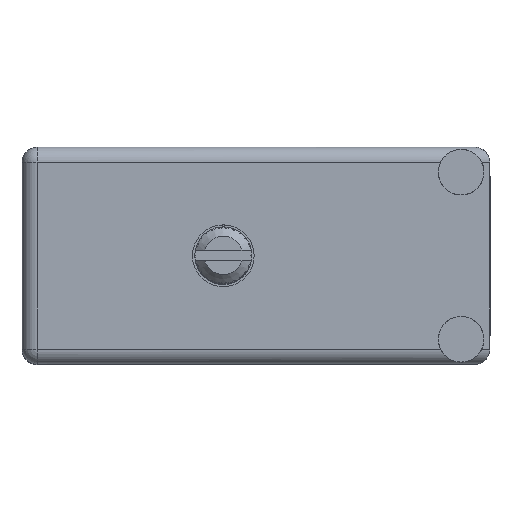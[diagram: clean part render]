
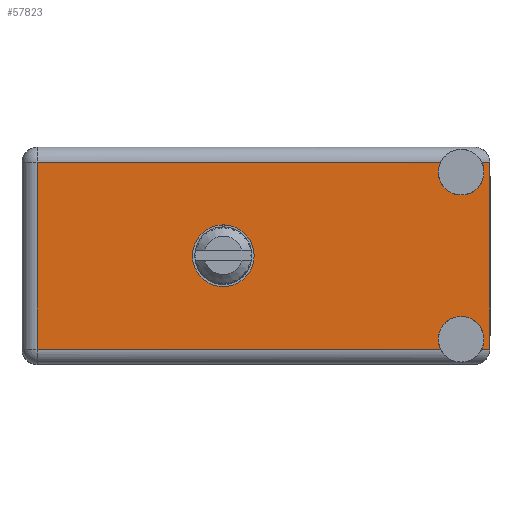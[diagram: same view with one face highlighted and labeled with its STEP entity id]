
A CAD part, top view. The second image highlights one B-rep face of the part: STEP entity #57823.
In plain terms, the highlighted face is planar.
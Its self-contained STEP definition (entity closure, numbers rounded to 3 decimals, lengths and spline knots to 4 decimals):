
#1668 = VECTOR ( 'NONE', #64394, 39.3701 ) ;
#2582 = ORIENTED_EDGE ( 'NONE', *, *, #130033, .F. ) ;
#2825 = CARTESIAN_POINT ( 'NONE',  ( 0.6625, 0.906, -0.3575 ) ) ;
#3331 = VERTEX_POINT ( 'NONE', #7955 ) ;
#4604 = ORIENTED_EDGE ( 'NONE', *, *, #117430, .T. ) ;
#6248 = VERTEX_POINT ( 'NONE', #70813 ) ;
#6480 = LINE ( 'NONE', #102697, #18150 ) ;
#7955 = CARTESIAN_POINT ( 'NONE',  ( 1.445, 0.906, -0.1575 ) ) ;
#9288 = LINE ( 'NONE', #59243, #58652 ) ;
#10315 = VERTEX_POINT ( 'NONE', #190705 ) ;
#10355 = CARTESIAN_POINT ( 'NONE',  ( 1.445, 0.906, -0.6325 ) ) ;
#11367 = VECTOR ( 'NONE', #15584, 39.3701 ) ;
#11597 = CARTESIAN_POINT ( 'NONE',  ( 1.3774, 0.906, -0.05 ) ) ;
#15584 = DIRECTION ( 'NONE',  ( 0., 0., 1. ) ) ;
#17100 = EDGE_CURVE ( 'NONE', #79199, #106583, #9288, .T. ) ;
#18150 = VECTOR ( 'NONE', #28124, 39.3701 ) ;
#18430 = ORIENTED_EDGE ( 'NONE', *, *, #21347, .F. ) ;
#21159 = CARTESIAN_POINT ( 'NONE',  ( 1.445, 0.906, -0.6325 ) ) ;
#21347 = EDGE_CURVE ( 'NONE', #79199, #6248, #82031, .T. ) ;
#26795 = DIRECTION ( 'NONE',  ( 0., 0., 1. ) ) ;
#28124 = DIRECTION ( 'NONE',  ( -1., 0., 0. ) ) ;
#29673 = AXIS2_PLACEMENT_3D ( 'NONE', #10355, #70163, #129662 ) ;
#37253 = EDGE_LOOP ( 'NONE', ( #142468, #139197 ) ) ;
#40499 = CIRCLE ( 'NONE', #71607, 0.075 ) ;
#41584 = VERTEX_POINT ( 'NONE', #65179 ) ;
#42517 = EDGE_CURVE ( 'NONE', #167241, #119506, #142861, .T. ) ;
#46506 = PLANE ( 'NONE',  #102972 ) ;
#54446 = CARTESIAN_POINT ( 'NONE',  ( 0.6625, 0.906, -0.256 ) ) ;
#55067 = AXIS2_PLACEMENT_3D ( 'NONE', #156459, #128154, #82593 ) ;
#57823 = ADVANCED_FACE ( 'NONE', ( #85024, #117999 ), #46506, .T. ) ;
#58652 = VECTOR ( 'NONE', #162889, 39.3701 ) ;
#59243 = CARTESIAN_POINT ( 'NONE',  ( 0., 0.906, -0.665 ) ) ;
#60384 = LINE ( 'NONE', #154798, #1668 ) ;
#60648 = EDGE_CURVE ( 'NONE', #3331, #182583, #40499, .T. ) ;
#64394 = DIRECTION ( 'NONE',  ( 0., 0., 1. ) ) ;
#64569 = DIRECTION ( 'NONE',  ( 0., 0., 1. ) ) ;
#65179 = CARTESIAN_POINT ( 'NONE',  ( 1.5126, 0.906, -0.05 ) ) ;
#70163 = DIRECTION ( 'NONE',  ( 0., 1., 0. ) ) ;
#70813 = CARTESIAN_POINT ( 'NONE',  ( 1.539, 0.906, -0.05 ) ) ;
#71607 = AXIS2_PLACEMENT_3D ( 'NONE', #116549, #192265, #26795 ) ;
#79199 = VERTEX_POINT ( 'NONE', #116572 ) ;
#79901 = ORIENTED_EDGE ( 'NONE', *, *, #189467, .T. ) ;
#81766 = CIRCLE ( 'NONE', #163083, 0.1015 ) ;
#82031 = LINE ( 'NONE', #150661, #11367 ) ;
#82593 = DIRECTION ( 'NONE',  ( 0., 0., 1. ) ) ;
#83786 = ORIENTED_EDGE ( 'NONE', *, *, #60648, .F. ) ;
#85024 = FACE_BOUND ( 'NONE', #37253, .T. ) ;
#88474 = AXIS2_PLACEMENT_3D ( 'NONE', #21159, #154968, #64569 ) ;
#88732 = CARTESIAN_POINT ( 'NONE',  ( 1.539, 0.906, -0.05 ) ) ;
#88858 = CARTESIAN_POINT ( 'NONE',  ( 0.05, 0.906, -0.665 ) ) ;
#89525 = CIRCLE ( 'NONE', #29673, 0.075 ) ;
#90859 = DIRECTION ( 'NONE',  ( 0., 0., 1. ) ) ;
#91681 = VERTEX_POINT ( 'NONE', #181531 ) ;
#93095 = CIRCLE ( 'NONE', #88474, 0.075 ) ;
#94346 = DIRECTION ( 'NONE',  ( 0., 1., 0. ) ) ;
#96861 = VERTEX_POINT ( 'NONE', #104162 ) ;
#98959 = ORIENTED_EDGE ( 'NONE', *, *, #169520, .T. ) ;
#102697 = CARTESIAN_POINT ( 'NONE',  ( 0., 0.906, -0.665 ) ) ;
#102972 = AXIS2_PLACEMENT_3D ( 'NONE', #165993, #181079, #90859 ) ;
#104162 = CARTESIAN_POINT ( 'NONE',  ( 0.05, 0.906, -0.05 ) ) ;
#104633 = CARTESIAN_POINT ( 'NONE',  ( 0.6625, 0.906, -0.459 ) ) ;
#106583 = VERTEX_POINT ( 'NONE', #138663 ) ;
#108004 = ORIENTED_EDGE ( 'NONE', *, *, #190427, .F. ) ;
#113003 = EDGE_LOOP ( 'NONE', ( #98959, #83786, #2582, #79901, #18430, #158748, #108004, #120141, #4604, #118377 ) ) ;
#116549 = CARTESIAN_POINT ( 'NONE',  ( 1.445, 0.906, -0.0825 ) ) ;
#116572 = CARTESIAN_POINT ( 'NONE',  ( 1.539, 0.906, -0.665 ) ) ;
#117430 = EDGE_CURVE ( 'NONE', #10315, #151895, #6480, .T. ) ;
#117999 = FACE_OUTER_BOUND ( 'NONE', #113003, .T. ) ;
#118377 = ORIENTED_EDGE ( 'NONE', *, *, #157691, .T. ) ;
#119506 = VERTEX_POINT ( 'NONE', #104633 ) ;
#120141 = ORIENTED_EDGE ( 'NONE', *, *, #177153, .F. ) ;
#122569 = CIRCLE ( 'NONE', #55067, 0.075 ) ;
#127330 = LINE ( 'NONE', #181764, #176738 ) ;
#128154 = DIRECTION ( 'NONE',  ( 0., 1., 0. ) ) ;
#129662 = DIRECTION ( 'NONE',  ( 0., 0., 1. ) ) ;
#130033 = EDGE_CURVE ( 'NONE', #41584, #3331, #122569, .T. ) ;
#132489 = AXIS2_PLACEMENT_3D ( 'NONE', #168722, #183804, #184454 ) ;
#135081 = DIRECTION ( 'NONE',  ( 1., 0., 0. ) ) ;
#138663 = CARTESIAN_POINT ( 'NONE',  ( 1.5126, 0.906, -0.665 ) ) ;
#139197 = ORIENTED_EDGE ( 'NONE', *, *, #194499, .F. ) ;
#142468 = ORIENTED_EDGE ( 'NONE', *, *, #42517, .F. ) ;
#142861 = CIRCLE ( 'NONE', #132489, 0.1015 ) ;
#146285 = LINE ( 'NONE', #88732, #179333 ) ;
#149381 = DIRECTION ( 'NONE',  ( 1., 0., 0. ) ) ;
#150661 = CARTESIAN_POINT ( 'NONE',  ( 1.539, 0.906, 0. ) ) ;
#151895 = VERTEX_POINT ( 'NONE', #88858 ) ;
#154798 = CARTESIAN_POINT ( 'NONE',  ( 0.05, 0.906, -0.715 ) ) ;
#154968 = DIRECTION ( 'NONE',  ( 0., 1., 0. ) ) ;
#156459 = CARTESIAN_POINT ( 'NONE',  ( 1.445, 0.906, -0.0825 ) ) ;
#157691 = EDGE_CURVE ( 'NONE', #151895, #96861, #60384, .T. ) ;
#158748 = ORIENTED_EDGE ( 'NONE', *, *, #17100, .T. ) ;
#162889 = DIRECTION ( 'NONE',  ( -1., 0., 0. ) ) ;
#163083 = AXIS2_PLACEMENT_3D ( 'NONE', #2825, #94346, #170055 ) ;
#165993 = CARTESIAN_POINT ( 'NONE',  ( 0., 0.906, -0.715 ) ) ;
#167241 = VERTEX_POINT ( 'NONE', #54446 ) ;
#168722 = CARTESIAN_POINT ( 'NONE',  ( 0.6625, 0.906, -0.3575 ) ) ;
#169520 = EDGE_CURVE ( 'NONE', #96861, #182583, #127330, .T. ) ;
#170055 = DIRECTION ( 'NONE',  ( 0., 0., 1. ) ) ;
#176738 = VECTOR ( 'NONE', #135081, 39.3701 ) ;
#177153 = EDGE_CURVE ( 'NONE', #10315, #91681, #93095, .T. ) ;
#179333 = VECTOR ( 'NONE', #149381, 39.3701 ) ;
#181079 = DIRECTION ( 'NONE',  ( 0., 1., 0. ) ) ;
#181531 = CARTESIAN_POINT ( 'NONE',  ( 1.445, 0.906, -0.5575 ) ) ;
#181764 = CARTESIAN_POINT ( 'NONE',  ( 1.539, 0.906, -0.05 ) ) ;
#182583 = VERTEX_POINT ( 'NONE', #11597 ) ;
#183804 = DIRECTION ( 'NONE',  ( 0., 1., 0. ) ) ;
#184454 = DIRECTION ( 'NONE',  ( 0., 0., 1. ) ) ;
#189467 = EDGE_CURVE ( 'NONE', #41584, #6248, #146285, .T. ) ;
#190427 = EDGE_CURVE ( 'NONE', #91681, #106583, #89525, .T. ) ;
#190705 = CARTESIAN_POINT ( 'NONE',  ( 1.3774, 0.906, -0.665 ) ) ;
#192265 = DIRECTION ( 'NONE',  ( 0., 1., 0. ) ) ;
#194499 = EDGE_CURVE ( 'NONE', #119506, #167241, #81766, .T. ) ;
